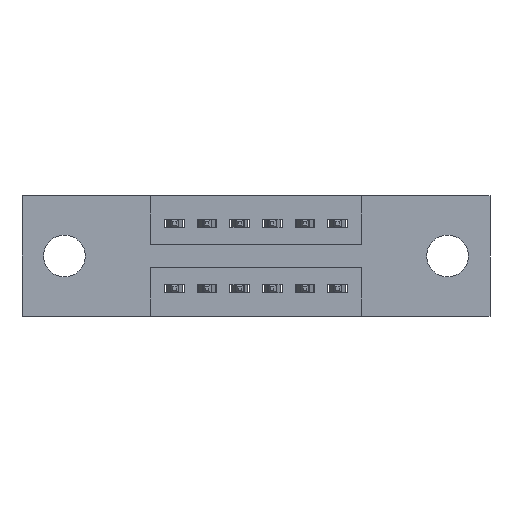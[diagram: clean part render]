
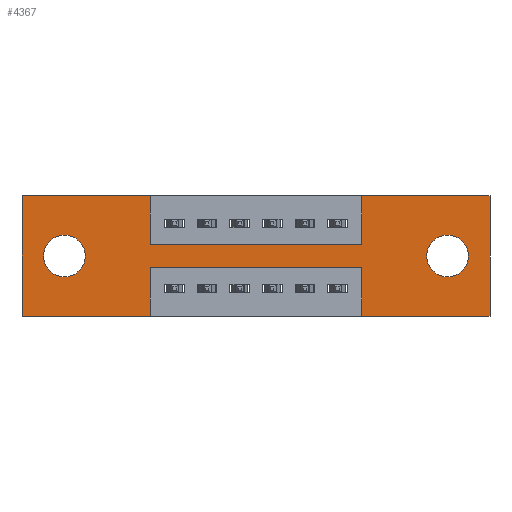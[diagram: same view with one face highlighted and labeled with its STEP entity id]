
A CAD part, front view. The second image highlights one B-rep face of the part: STEP entity #4367.
In plain terms, the highlighted planar face has unit normal (0, -1, 0).
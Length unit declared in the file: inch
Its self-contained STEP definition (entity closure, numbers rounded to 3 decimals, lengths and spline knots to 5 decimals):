
#27 = CARTESIAN_POINT ( 'NONE',  ( 0.3925, 0., -0.15 ) ) ;
#30 = VERTEX_POINT ( 'NONE', #5339 ) ;
#65 = VERTEX_POINT ( 'NONE', #2607 ) ;
#70 = EDGE_CURVE ( 'NONE', #30, #2601, #6525, .T. ) ;
#381 = ORIENTED_EDGE ( 'NONE', *, *, #7277, .T. ) ;
#638 = CARTESIAN_POINT ( 'NONE',  ( 0., 0., -0.37 ) ) ;
#686 = ORIENTED_EDGE ( 'NONE', *, *, #1303, .F. ) ;
#747 = VECTOR ( 'NONE', #9265, 39.37008 ) ;
#788 = CARTESIAN_POINT ( 'NONE',  ( 0.13, 0., -0.185 ) ) ;
#836 = DIRECTION ( 'NONE',  ( 0., 0., 1. ) ) ;
#1303 = EDGE_CURVE ( 'NONE', #5949, #7385, #9509, .T. ) ;
#1384 = VERTEX_POINT ( 'NONE', #3651 ) ;
#1561 = PLANE ( 'NONE',  #5519 ) ;
#1643 = DIRECTION ( 'NONE',  ( 0., 0., 1. ) ) ;
#1721 = DIRECTION ( 'NONE',  ( 0., 0., 1. ) ) ;
#1728 = CARTESIAN_POINT ( 'NONE',  ( 0., 0., -0.37 ) ) ;
#1734 = CARTESIAN_POINT ( 'NONE',  ( 1.435, 0., 0. ) ) ;
#1758 = VERTEX_POINT ( 'NONE', #6138 ) ;
#1760 = DIRECTION ( 'NONE',  ( 0., 0., -1. ) ) ;
#1765 = DIRECTION ( 'NONE',  ( 0., 0., -1. ) ) ;
#1766 = EDGE_LOOP ( 'NONE', ( #381, #5831 ) ) ;
#1878 = CARTESIAN_POINT ( 'NONE',  ( 0., 0., -0.37 ) ) ;
#1900 = VECTOR ( 'NONE', #1760, 39.37008 ) ;
#1961 = ORIENTED_EDGE ( 'NONE', *, *, #3108, .F. ) ;
#2199 = VERTEX_POINT ( 'NONE', #5080 ) ;
#2353 = EDGE_CURVE ( 'NONE', #65, #5949, #6718, .T. ) ;
#2412 = VECTOR ( 'NONE', #7456, 39.37008 ) ;
#2429 = LINE ( 'NONE', #3506, #9159 ) ;
#2474 = VERTEX_POINT ( 'NONE', #1878 ) ;
#2478 = LINE ( 'NONE', #9212, #7506 ) ;
#2536 = VERTEX_POINT ( 'NONE', #27 ) ;
#2601 = VERTEX_POINT ( 'NONE', #9148 ) ;
#2604 = EDGE_LOOP ( 'NONE', ( #9198, #9468, #8371, #8575, #5545, #686, #2845, #1961, #7169, #7389, #4869, #7295 ) ) ;
#2607 = CARTESIAN_POINT ( 'NONE',  ( 1.0425, 0., -0.15 ) ) ;
#2642 = DIRECTION ( 'NONE',  ( 0., 1., 0. ) ) ;
#2684 = VECTOR ( 'NONE', #3468, 39.37008 ) ;
#2845 = ORIENTED_EDGE ( 'NONE', *, *, #2353, .F. ) ;
#2953 = CARTESIAN_POINT ( 'NONE',  ( 1.0425, 0., 0. ) ) ;
#3081 = EDGE_CURVE ( 'NONE', #8141, #9290, #3771, .T. ) ;
#3108 = EDGE_CURVE ( 'NONE', #2536, #65, #3528, .T. ) ;
#3134 = CARTESIAN_POINT ( 'NONE',  ( 1.0425, 0., 0. ) ) ;
#3182 = AXIS2_PLACEMENT_3D ( 'NONE', #788, #6334, #1643 ) ;
#3297 = ORIENTED_EDGE ( 'NONE', *, *, #7473, .T. ) ;
#3375 = CARTESIAN_POINT ( 'NONE',  ( 0.3925, 0., -0.37 ) ) ;
#3468 = DIRECTION ( 'NONE',  ( -1., 0., 0. ) ) ;
#3506 = CARTESIAN_POINT ( 'NONE',  ( 1.435, 0., 0. ) ) ;
#3528 = LINE ( 'NONE', #8751, #5613 ) ;
#3574 = CARTESIAN_POINT ( 'NONE',  ( 0., 0., 0. ) ) ;
#3651 = CARTESIAN_POINT ( 'NONE',  ( 0.3925, 0., 0. ) ) ;
#3684 = VERTEX_POINT ( 'NONE', #4777 ) ;
#3771 = LINE ( 'NONE', #638, #9306 ) ;
#3793 = EDGE_CURVE ( 'NONE', #2474, #7857, #2478, .T. ) ;
#3838 = CARTESIAN_POINT ( 'NONE',  ( 0., 0., 0. ) ) ;
#3937 = CIRCLE ( 'NONE', #9133, 0.064 ) ;
#4015 = CARTESIAN_POINT ( 'NONE',  ( 1.0425, 0., -0.37 ) ) ;
#4031 = AXIS2_PLACEMENT_3D ( 'NONE', #8853, #4812, #9484 ) ;
#4271 = CARTESIAN_POINT ( 'NONE',  ( 0.13, 0., -0.185 ) ) ;
#4293 = LINE ( 'NONE', #8989, #1900 ) ;
#4367 = ADVANCED_FACE ( 'NONE', ( #5355, #6992, #5120 ), #1561, .T. ) ;
#4720 = CARTESIAN_POINT ( 'NONE',  ( 0.13, 0., -0.121 ) ) ;
#4777 = CARTESIAN_POINT ( 'NONE',  ( 0.13, 0., -0.249 ) ) ;
#4812 = DIRECTION ( 'NONE',  ( 0., 1., 0. ) ) ;
#4832 = LINE ( 'NONE', #5452, #2412 ) ;
#4869 = ORIENTED_EDGE ( 'NONE', *, *, #3793, .F. ) ;
#4974 = DIRECTION ( 'NONE',  ( 1., 0., 0. ) ) ;
#5080 = CARTESIAN_POINT ( 'NONE',  ( 1.305, 0., -0.121 ) ) ;
#5093 = DIRECTION ( 'NONE',  ( 0., 0., 1. ) ) ;
#5120 = FACE_OUTER_BOUND ( 'NONE', #2604, .T. ) ;
#5339 = CARTESIAN_POINT ( 'NONE',  ( 1.0425, 0., -0.22 ) ) ;
#5355 = FACE_BOUND ( 'NONE', #1766, .T. ) ;
#5392 = EDGE_CURVE ( 'NONE', #8062, #2474, #6335, .T. ) ;
#5446 = EDGE_CURVE ( 'NONE', #7385, #8141, #2429, .T. ) ;
#5452 = CARTESIAN_POINT ( 'NONE',  ( 0.3925, 0., 0. ) ) ;
#5474 = CARTESIAN_POINT ( 'NONE',  ( 0., 0., 0. ) ) ;
#5519 = AXIS2_PLACEMENT_3D ( 'NONE', #1728, #7802, #1765 ) ;
#5545 = ORIENTED_EDGE ( 'NONE', *, *, #5446, .F. ) ;
#5613 = VECTOR ( 'NONE', #7026, 39.37008 ) ;
#5650 = CARTESIAN_POINT ( 'NONE',  ( 1.0425, 0., -0.37 ) ) ;
#5831 = ORIENTED_EDGE ( 'NONE', *, *, #7459, .T. ) ;
#5949 = VERTEX_POINT ( 'NONE', #3134 ) ;
#6138 = CARTESIAN_POINT ( 'NONE',  ( 1.305, 0., -0.249 ) ) ;
#6334 = DIRECTION ( 'NONE',  ( 0., 1., 0. ) ) ;
#6335 = LINE ( 'NONE', #7077, #2684 ) ;
#6463 = EDGE_CURVE ( 'NONE', #7857, #1384, #8937, .T. ) ;
#6492 = VECTOR ( 'NONE', #1721, 39.37008 ) ;
#6525 = LINE ( 'NONE', #9361, #747 ) ;
#6641 = EDGE_CURVE ( 'NONE', #3684, #8584, #9236, .T. ) ;
#6681 = EDGE_CURVE ( 'NONE', #9290, #30, #7543, .T. ) ;
#6718 = LINE ( 'NONE', #2953, #6492 ) ;
#6930 = DIRECTION ( 'NONE',  ( -1., 0., 0. ) ) ;
#6992 = FACE_BOUND ( 'NONE', #8491, .T. ) ;
#7026 = DIRECTION ( 'NONE',  ( 1., 0., 0. ) ) ;
#7077 = CARTESIAN_POINT ( 'NONE',  ( 0., 0., -0.37 ) ) ;
#7169 = ORIENTED_EDGE ( 'NONE', *, *, #7181, .F. ) ;
#7172 = CARTESIAN_POINT ( 'NONE',  ( 1.305, 0., -0.185 ) ) ;
#7181 = EDGE_CURVE ( 'NONE', #1384, #2536, #4832, .T. ) ;
#7277 = EDGE_CURVE ( 'NONE', #2199, #1758, #9149, .T. ) ;
#7295 = ORIENTED_EDGE ( 'NONE', *, *, #5392, .F. ) ;
#7385 = VERTEX_POINT ( 'NONE', #1734 ) ;
#7389 = ORIENTED_EDGE ( 'NONE', *, *, #6463, .F. ) ;
#7456 = DIRECTION ( 'NONE',  ( 0., 0., -1. ) ) ;
#7459 = EDGE_CURVE ( 'NONE', #1758, #2199, #3937, .T. ) ;
#7473 = EDGE_CURVE ( 'NONE', #8584, #3684, #7741, .T. ) ;
#7506 = VECTOR ( 'NONE', #8997, 39.37008 ) ;
#7543 = LINE ( 'NONE', #5650, #9042 ) ;
#7605 = ORIENTED_EDGE ( 'NONE', *, *, #6641, .T. ) ;
#7741 = CIRCLE ( 'NONE', #9532, 0.064 ) ;
#7797 = DIRECTION ( 'NONE',  ( 0., 0., -1. ) ) ;
#7802 = DIRECTION ( 'NONE',  ( 0., -1., 0. ) ) ;
#7857 = VERTEX_POINT ( 'NONE', #5474 ) ;
#7983 = DIRECTION ( 'NONE',  ( 0., 0., -1. ) ) ;
#8062 = VERTEX_POINT ( 'NONE', #3375 ) ;
#8084 = EDGE_CURVE ( 'NONE', #2601, #8062, #4293, .T. ) ;
#8141 = VERTEX_POINT ( 'NONE', #9050 ) ;
#8371 = ORIENTED_EDGE ( 'NONE', *, *, #6681, .F. ) ;
#8491 = EDGE_LOOP ( 'NONE', ( #3297, #7605 ) ) ;
#8575 = ORIENTED_EDGE ( 'NONE', *, *, #3081, .F. ) ;
#8584 = VERTEX_POINT ( 'NONE', #4720 ) ;
#8729 = VECTOR ( 'NONE', #9364, 39.37008 ) ;
#8751 = CARTESIAN_POINT ( 'NONE',  ( 0.3925, 0., -0.15 ) ) ;
#8853 = CARTESIAN_POINT ( 'NONE',  ( 1.305, 0., -0.185 ) ) ;
#8937 = LINE ( 'NONE', #3838, #8729 ) ;
#8989 = CARTESIAN_POINT ( 'NONE',  ( 0.3925, 0., -0.37 ) ) ;
#8997 = DIRECTION ( 'NONE',  ( 0., 0., 1. ) ) ;
#9042 = VECTOR ( 'NONE', #836, 39.37008 ) ;
#9050 = CARTESIAN_POINT ( 'NONE',  ( 1.435, 0., -0.37 ) ) ;
#9080 = DIRECTION ( 'NONE',  ( 0., 1., 0. ) ) ;
#9133 = AXIS2_PLACEMENT_3D ( 'NONE', #7172, #2642, #7797 ) ;
#9148 = CARTESIAN_POINT ( 'NONE',  ( 0.3925, 0., -0.22 ) ) ;
#9149 = CIRCLE ( 'NONE', #4031, 0.064 ) ;
#9159 = VECTOR ( 'NONE', #7983, 39.37008 ) ;
#9198 = ORIENTED_EDGE ( 'NONE', *, *, #8084, .F. ) ;
#9212 = CARTESIAN_POINT ( 'NONE',  ( 0., 0., 0. ) ) ;
#9236 = CIRCLE ( 'NONE', #3182, 0.064 ) ;
#9265 = DIRECTION ( 'NONE',  ( -1., 0., 0. ) ) ;
#9290 = VERTEX_POINT ( 'NONE', #4015 ) ;
#9306 = VECTOR ( 'NONE', #6930, 39.37008 ) ;
#9331 = VECTOR ( 'NONE', #4974, 39.37008 ) ;
#9361 = CARTESIAN_POINT ( 'NONE',  ( 0.3925, 0., -0.22 ) ) ;
#9364 = DIRECTION ( 'NONE',  ( 1., 0., 0. ) ) ;
#9468 = ORIENTED_EDGE ( 'NONE', *, *, #70, .F. ) ;
#9484 = DIRECTION ( 'NONE',  ( 0., 0., -1. ) ) ;
#9509 = LINE ( 'NONE', #3574, #9331 ) ;
#9532 = AXIS2_PLACEMENT_3D ( 'NONE', #4271, #9080, #5093 ) ;
